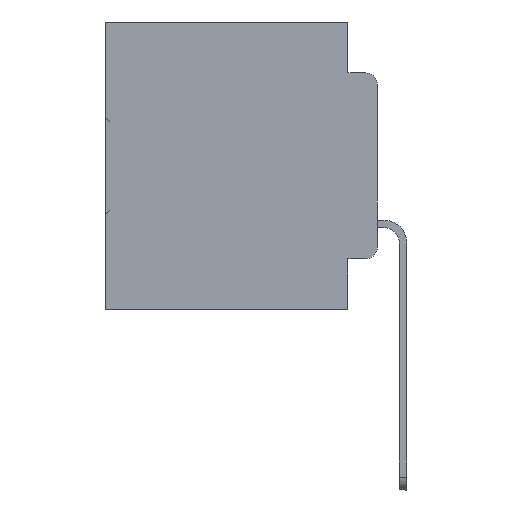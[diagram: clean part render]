
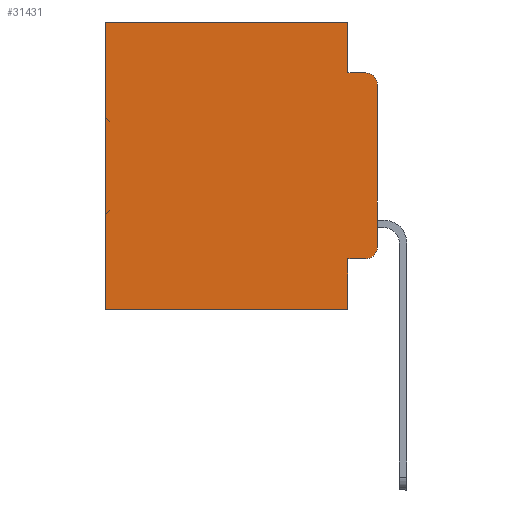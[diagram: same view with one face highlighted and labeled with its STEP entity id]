
A CAD part, left-side view. The second image highlights one B-rep face of the part: STEP entity #31431.
In plain terms, the highlighted planar face has unit normal (-1, 0, 0).
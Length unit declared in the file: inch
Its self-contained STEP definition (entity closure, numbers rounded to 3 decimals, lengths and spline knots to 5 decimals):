
#47 = CARTESIAN_POINT ( 'NONE',  ( 0.298, 0., 0. ) ) ;
#1184 = CARTESIAN_POINT ( 'NONE',  ( 0.298, 0.051, -0.0885 ) ) ;
#1243 = ORIENTED_EDGE ( 'NONE', *, *, #19961, .T. ) ;
#1292 = CARTESIAN_POINT ( 'NONE',  ( 0.298, 0.051, -0.5 ) ) ;
#1339 = LINE ( 'NONE', #30404, #17652 ) ;
#1402 = DIRECTION ( 'NONE',  ( 0., 0., -1. ) ) ;
#1570 = ORIENTED_EDGE ( 'NONE', *, *, #8525, .F. ) ;
#1603 = VERTEX_POINT ( 'NONE', #5491 ) ;
#2078 = EDGE_CURVE ( 'NONE', #29274, #18737, #10763, .T. ) ;
#2566 = DIRECTION ( 'NONE',  ( 0., 0., -1. ) ) ;
#2828 = CARTESIAN_POINT ( 'NONE',  ( 0.298, 0.473, 0. ) ) ;
#3349 = EDGE_CURVE ( 'NONE', #26922, #13881, #18433, .T. ) ;
#3512 = EDGE_CURVE ( 'NONE', #31738, #25198, #20108, .T. ) ;
#3554 = AXIS2_PLACEMENT_3D ( 'NONE', #5263, #28270, #5445 ) ;
#4379 = CIRCLE ( 'NONE', #4975, 0.02 ) ;
#4975 = AXIS2_PLACEMENT_3D ( 'NONE', #18261, #29787, #10703 ) ;
#5263 = CARTESIAN_POINT ( 'NONE',  ( 0.298, 0.02, -0.1085 ) ) ;
#5347 = CARTESIAN_POINT ( 'NONE',  ( 0.298, 0.02, -0.0885 ) ) ;
#5419 = LINE ( 'NONE', #8972, #26732 ) ;
#5445 = DIRECTION ( 'NONE',  ( 0., 0., -1. ) ) ;
#5491 = CARTESIAN_POINT ( 'NONE',  ( 0.298, 0.473, 0. ) ) ;
#8479 = LINE ( 'NONE', #2828, #35750 ) ;
#8525 = EDGE_CURVE ( 'NONE', #25198, #18737, #5419, .T. ) ;
#8972 = CARTESIAN_POINT ( 'NONE',  ( 0.298, 0.051, -0.0885 ) ) ;
#10634 = PLANE ( 'NONE',  #23917 ) ;
#10703 = DIRECTION ( 'NONE',  ( 0., 0., -1. ) ) ;
#10763 = CIRCLE ( 'NONE', #3554, 0.02 ) ;
#11998 = DIRECTION ( 'NONE',  ( 0., -1., 0. ) ) ;
#12275 = VERTEX_POINT ( 'NONE', #31872 ) ;
#12464 = CARTESIAN_POINT ( 'NONE',  ( 0.298, 0.051, -0.4115 ) ) ;
#12843 = DIRECTION ( 'NONE',  ( 0., 0., -1. ) ) ;
#13881 = VERTEX_POINT ( 'NONE', #35721 ) ;
#14380 = LINE ( 'NONE', #47, #15717 ) ;
#15717 = VECTOR ( 'NONE', #31202, 39.37008 ) ;
#16994 = ORIENTED_EDGE ( 'NONE', *, *, #23631, .F. ) ;
#17350 = DIRECTION ( 'NONE',  ( 0., 1., 0. ) ) ;
#17652 = VECTOR ( 'NONE', #12843, 39.37008 ) ;
#18073 = VERTEX_POINT ( 'NONE', #35226 ) ;
#18081 = VECTOR ( 'NONE', #2566, 39.37008 ) ;
#18261 = CARTESIAN_POINT ( 'NONE',  ( 0.298, 0.02, -0.3915 ) ) ;
#18433 = LINE ( 'NONE', #29953, #24725 ) ;
#18737 = VERTEX_POINT ( 'NONE', #5347 ) ;
#18759 = FACE_OUTER_BOUND ( 'NONE', #19173, .T. ) ;
#19173 = EDGE_LOOP ( 'NONE', ( #16994, #21669, #1570, #32829, #1243, #36794, #36586, #33379, #34611, #22805 ) ) ;
#19501 = CARTESIAN_POINT ( 'NONE',  ( 0.298, 0., 0. ) ) ;
#19814 = CARTESIAN_POINT ( 'NONE',  ( 0.298, 0., -0.5 ) ) ;
#19961 = EDGE_CURVE ( 'NONE', #31738, #1603, #14380, .T. ) ;
#19986 = VECTOR ( 'NONE', #21005, 39.37008 ) ;
#20108 = LINE ( 'NONE', #28232, #18081 ) ;
#21005 = DIRECTION ( 'NONE',  ( 0., 0., -1. ) ) ;
#21669 = ORIENTED_EDGE ( 'NONE', *, *, #2078, .T. ) ;
#22093 = DIRECTION ( 'NONE',  ( 0., 0., -1. ) ) ;
#22155 = DIRECTION ( 'NONE',  ( 1., 0., 0. ) ) ;
#22805 = ORIENTED_EDGE ( 'NONE', *, *, #25613, .T. ) ;
#23631 = EDGE_CURVE ( 'NONE', #29274, #12275, #1339, .T. ) ;
#23917 = AXIS2_PLACEMENT_3D ( 'NONE', #19501, #22155, #1402 ) ;
#24031 = VERTEX_POINT ( 'NONE', #1292 ) ;
#24725 = VECTOR ( 'NONE', #30523, 39.37008 ) ;
#25036 = EDGE_CURVE ( 'NONE', #24031, #18073, #34176, .T. ) ;
#25065 = EDGE_CURVE ( 'NONE', #26922, #24031, #25661, .T. ) ;
#25198 = VERTEX_POINT ( 'NONE', #1184 ) ;
#25613 = EDGE_CURVE ( 'NONE', #13881, #12275, #4379, .T. ) ;
#25661 = LINE ( 'NONE', #37188, #19986 ) ;
#26732 = VECTOR ( 'NONE', #11998, 39.37008 ) ;
#26922 = VERTEX_POINT ( 'NONE', #12464 ) ;
#28232 = CARTESIAN_POINT ( 'NONE',  ( 0.298, 0.051, 0. ) ) ;
#28270 = DIRECTION ( 'NONE',  ( -1., 0., 0. ) ) ;
#28335 = EDGE_CURVE ( 'NONE', #1603, #18073, #8479, .T. ) ;
#29274 = VERTEX_POINT ( 'NONE', #31102 ) ;
#29787 = DIRECTION ( 'NONE',  ( -1., 0., 0. ) ) ;
#29953 = CARTESIAN_POINT ( 'NONE',  ( 0.298, 0.051, -0.4115 ) ) ;
#30404 = CARTESIAN_POINT ( 'NONE',  ( 0.298, 0., 0. ) ) ;
#30523 = DIRECTION ( 'NONE',  ( 0., -1., 0. ) ) ;
#31102 = CARTESIAN_POINT ( 'NONE',  ( 0.298, 0., -0.1085 ) ) ;
#31202 = DIRECTION ( 'NONE',  ( 0., 1., 0. ) ) ;
#31431 = ADVANCED_FACE ( 'NONE', ( #18759 ), #10634, .F. ) ;
#31738 = VERTEX_POINT ( 'NONE', #36269 ) ;
#31872 = CARTESIAN_POINT ( 'NONE',  ( 0.298, 0., -0.3915 ) ) ;
#32829 = ORIENTED_EDGE ( 'NONE', *, *, #3512, .F. ) ;
#33379 = ORIENTED_EDGE ( 'NONE', *, *, #25065, .F. ) ;
#34176 = LINE ( 'NONE', #19814, #35054 ) ;
#34611 = ORIENTED_EDGE ( 'NONE', *, *, #3349, .T. ) ;
#35054 = VECTOR ( 'NONE', #17350, 39.37008 ) ;
#35226 = CARTESIAN_POINT ( 'NONE',  ( 0.298, 0.473, -0.5 ) ) ;
#35721 = CARTESIAN_POINT ( 'NONE',  ( 0.298, 0.02, -0.4115 ) ) ;
#35750 = VECTOR ( 'NONE', #22093, 39.37008 ) ;
#36269 = CARTESIAN_POINT ( 'NONE',  ( 0.298, 0.051, 0. ) ) ;
#36586 = ORIENTED_EDGE ( 'NONE', *, *, #25036, .F. ) ;
#36794 = ORIENTED_EDGE ( 'NONE', *, *, #28335, .T. ) ;
#37188 = CARTESIAN_POINT ( 'NONE',  ( 0.298, 0.051, 0. ) ) ;
